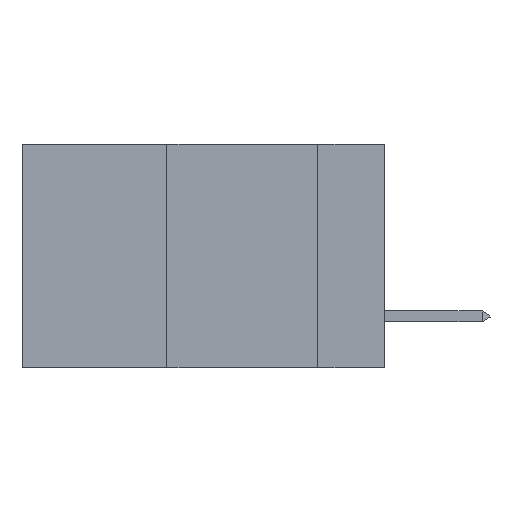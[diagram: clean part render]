
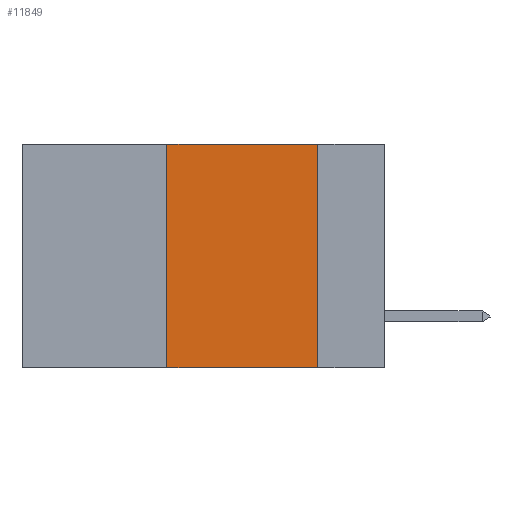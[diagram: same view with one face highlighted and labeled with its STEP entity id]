
A CAD part, left-side view. The second image highlights one B-rep face of the part: STEP entity #11849.
In plain terms, the highlighted planar face has unit normal (-1, 0, 0).
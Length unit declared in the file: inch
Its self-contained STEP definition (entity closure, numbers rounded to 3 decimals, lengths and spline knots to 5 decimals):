
#801 = CARTESIAN_POINT ( 'NONE',  ( 0., 0.6, 0. ) ) ;
#1128 = ORIENTED_EDGE ( 'NONE', *, *, #4933, .T. ) ;
#2291 = FACE_OUTER_BOUND ( 'NONE', #9077, .T. ) ;
#3380 = CARTESIAN_POINT ( 'NONE',  ( 0., 0.6, -0.37 ) ) ;
#3591 = DIRECTION ( 'NONE',  ( 0., -1., 0. ) ) ;
#4585 = LINE ( 'NONE', #14551, #11513 ) ;
#4778 = DIRECTION ( 'NONE',  ( 0., -1., 0. ) ) ;
#4933 = EDGE_CURVE ( 'NONE', #5826, #14679, #7762, .T. ) ;
#5295 = LINE ( 'NONE', #16211, #16380 ) ;
#5826 = VERTEX_POINT ( 'NONE', #6704 ) ;
#6443 = CARTESIAN_POINT ( 'NONE',  ( 0., 0.11, -0.37 ) ) ;
#6446 = CARTESIAN_POINT ( 'NONE',  ( 0., 0.36, 0. ) ) ;
#6704 = CARTESIAN_POINT ( 'NONE',  ( 0., 0.36, -0.37 ) ) ;
#6930 = ORIENTED_EDGE ( 'NONE', *, *, #9048, .F. ) ;
#7151 = AXIS2_PLACEMENT_3D ( 'NONE', #801, #9648, #9925 ) ;
#7762 = LINE ( 'NONE', #3380, #12480 ) ;
#8308 = CARTESIAN_POINT ( 'NONE',  ( 0., 0.11, 0. ) ) ;
#8385 = PLANE ( 'NONE',  #7151 ) ;
#8398 = VERTEX_POINT ( 'NONE', #8308 ) ;
#9048 = EDGE_CURVE ( 'NONE', #5826, #10411, #10600, .T. ) ;
#9077 = EDGE_LOOP ( 'NONE', ( #10680, #12965, #6930, #1128 ) ) ;
#9648 = DIRECTION ( 'NONE',  ( 1., 0., 0. ) ) ;
#9925 = DIRECTION ( 'NONE',  ( 0., 0., -1. ) ) ;
#10411 = VERTEX_POINT ( 'NONE', #13996 ) ;
#10600 = LINE ( 'NONE', #6446, #12562 ) ;
#10680 = ORIENTED_EDGE ( 'NONE', *, *, #14945, .F. ) ;
#11165 = EDGE_CURVE ( 'NONE', #10411, #8398, #5295, .T. ) ;
#11513 = VECTOR ( 'NONE', #14506, 39.37008 ) ;
#11849 = ADVANCED_FACE ( 'NONE', ( #2291 ), #8385, .F. ) ;
#12480 = VECTOR ( 'NONE', #4778, 39.37008 ) ;
#12562 = VECTOR ( 'NONE', #15526, 39.37008 ) ;
#12965 = ORIENTED_EDGE ( 'NONE', *, *, #11165, .F. ) ;
#13996 = CARTESIAN_POINT ( 'NONE',  ( 0., 0.36, 0. ) ) ;
#14506 = DIRECTION ( 'NONE',  ( 0., 0., -1. ) ) ;
#14551 = CARTESIAN_POINT ( 'NONE',  ( 0., 0.11, 0. ) ) ;
#14679 = VERTEX_POINT ( 'NONE', #6443 ) ;
#14945 = EDGE_CURVE ( 'NONE', #8398, #14679, #4585, .T. ) ;
#15526 = DIRECTION ( 'NONE',  ( 0., 0., 1. ) ) ;
#16211 = CARTESIAN_POINT ( 'NONE',  ( 0., 0.6, 0. ) ) ;
#16380 = VECTOR ( 'NONE', #3591, 39.37008 ) ;
